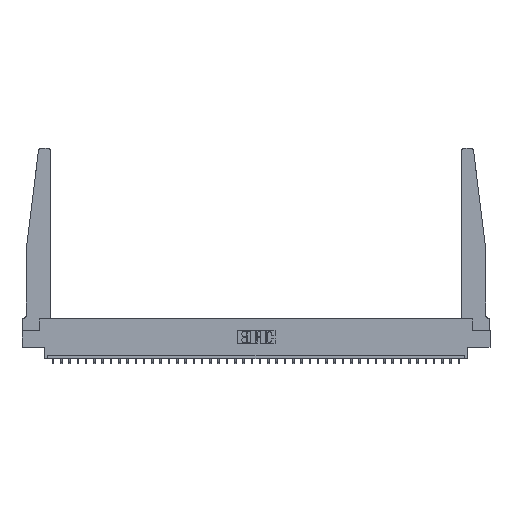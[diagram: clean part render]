
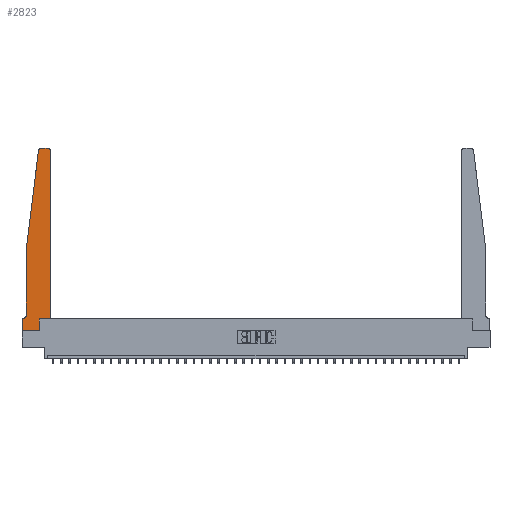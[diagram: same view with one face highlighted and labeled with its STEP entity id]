
A CAD part, top view. The second image highlights one B-rep face of the part: STEP entity #2823.
In plain terms, the highlighted planar face has unit normal (0, 0, 1).
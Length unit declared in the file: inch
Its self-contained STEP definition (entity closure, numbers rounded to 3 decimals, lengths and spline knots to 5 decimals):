
#106 = VERTEX_POINT ( 'NONE', #21183 ) ;
#502 = CARTESIAN_POINT ( 'NONE',  ( 0.2605, 0., 0.37 ) ) ;
#617 = ORIENTED_EDGE ( 'NONE', *, *, #6288, .T. ) ;
#631 = LINE ( 'NONE', #19562, #21369 ) ;
#884 = VECTOR ( 'NONE', #17345, 39.37008 ) ;
#1055 = CARTESIAN_POINT ( 'NONE',  ( 0.2605, 0.18, 0.37 ) ) ;
#1142 = ORIENTED_EDGE ( 'NONE', *, *, #24729, .T. ) ;
#1410 = CARTESIAN_POINT ( 'NONE',  ( 0.25, 2.75, 0.37 ) ) ;
#1413 = VECTOR ( 'NONE', #12961, 39.37008 ) ;
#2285 = ORIENTED_EDGE ( 'NONE', *, *, #34943, .T. ) ;
#2823 = ADVANCED_FACE ( 'NONE', ( #4828 ), #4085, .T. ) ;
#2883 = EDGE_CURVE ( 'NONE', #24931, #31924, #31074, .T. ) ;
#3437 = EDGE_CURVE ( 'NONE', #21624, #19020, #34818, .T. ) ;
#4085 = PLANE ( 'NONE',  #16069 ) ;
#4260 = VERTEX_POINT ( 'NONE', #10631 ) ;
#4573 = CARTESIAN_POINT ( 'NONE',  ( 0.065, 1.25, 0.37 ) ) ;
#4828 = FACE_OUTER_BOUND ( 'NONE', #7690, .T. ) ;
#5713 = VECTOR ( 'NONE', #20335, 39.37008 ) ;
#6008 = AXIS2_PLACEMENT_3D ( 'NONE', #9923, #28837, #12650 ) ;
#6239 = ORIENTED_EDGE ( 'NONE', *, *, #30972, .T. ) ;
#6288 = EDGE_CURVE ( 'NONE', #31924, #32049, #16930, .T. ) ;
#7283 = DIRECTION ( 'NONE',  ( -0.122, -0.992, 0. ) ) ;
#7435 = AXIS2_PLACEMENT_3D ( 'NONE', #12800, #31715, #15513 ) ;
#7573 = ORIENTED_EDGE ( 'NONE', *, *, #24124, .T. ) ;
#7690 = EDGE_LOOP ( 'NONE', ( #17055, #8442, #12728, #23685, #7573, #6239, #21444, #23729, #617, #2285, #1142, #27876 ) ) ;
#7839 = AXIS2_PLACEMENT_3D ( 'NONE', #31916, #15717, #34592 ) ;
#8350 = DIRECTION ( 'NONE',  ( -1., 0., 0. ) ) ;
#8442 = ORIENTED_EDGE ( 'NONE', *, *, #3437, .T. ) ;
#8556 = LINE ( 'NONE', #18305, #1413 ) ;
#8745 = DIRECTION ( 'NONE',  ( 0., -1., 0. ) ) ;
#9923 = CARTESIAN_POINT ( 'NONE',  ( 0.015, 0.2375, 0.37 ) ) ;
#10631 = CARTESIAN_POINT ( 'NONE',  ( 0.065, 0.2375, 0.37 ) ) ;
#11408 = LINE ( 'NONE', #24056, #18614 ) ;
#12240 = DIRECTION ( 'NONE',  ( 1., 0., 0. ) ) ;
#12650 = DIRECTION ( 'NONE',  ( -1., 0., 0. ) ) ;
#12728 = ORIENTED_EDGE ( 'NONE', *, *, #22366, .T. ) ;
#12782 = VERTEX_POINT ( 'NONE', #22865 ) ;
#12800 = CARTESIAN_POINT ( 'NONE',  ( 0.27653, 2.72, 0.37 ) ) ;
#12961 = DIRECTION ( 'NONE',  ( 0., 1., 0. ) ) ;
#13389 = LINE ( 'NONE', #32881, #21485 ) ;
#13698 = CIRCLE ( 'NONE', #7839, 0.03 ) ;
#14226 = CARTESIAN_POINT ( 'NONE',  ( 0., 0., 0.37 ) ) ;
#14302 = VERTEX_POINT ( 'NONE', #27363 ) ;
#15513 = DIRECTION ( 'NONE',  ( 1., 0., 0. ) ) ;
#15544 = LINE ( 'NONE', #4573, #28245 ) ;
#15635 = VERTEX_POINT ( 'NONE', #25544 ) ;
#15717 = DIRECTION ( 'NONE',  ( 0., 0., 1. ) ) ;
#15870 = LINE ( 'NONE', #24571, #30239 ) ;
#16069 = AXIS2_PLACEMENT_3D ( 'NONE', #23030, #28447, #12240 ) ;
#16695 = DIRECTION ( 'NONE',  ( 0., -1., 0. ) ) ;
#16930 = LINE ( 'NONE', #33522, #884 ) ;
#17055 = ORIENTED_EDGE ( 'NONE', *, *, #18005, .T. ) ;
#17345 = DIRECTION ( 'NONE',  ( 0., 1., 0. ) ) ;
#18005 = EDGE_CURVE ( 'NONE', #106, #21624, #18450, .T. ) ;
#18305 = CARTESIAN_POINT ( 'NONE',  ( 0.425, 0.18, 0.37 ) ) ;
#18450 = LINE ( 'NONE', #1410, #5713 ) ;
#18614 = VECTOR ( 'NONE', #34869, 39.37008 ) ;
#18995 = EDGE_CURVE ( 'NONE', #15635, #24931, #631, .T. ) ;
#19020 = VERTEX_POINT ( 'NONE', #22400 ) ;
#19562 = CARTESIAN_POINT ( 'NONE',  ( 0., 0., 0.37 ) ) ;
#20335 = DIRECTION ( 'NONE',  ( -1., 0., 0. ) ) ;
#21183 = CARTESIAN_POINT ( 'NONE',  ( 0.395, 2.75, 0.37 ) ) ;
#21369 = VECTOR ( 'NONE', #8745, 39.37008 ) ;
#21444 = ORIENTED_EDGE ( 'NONE', *, *, #18995, .T. ) ;
#21485 = VECTOR ( 'NONE', #16695, 39.37008 ) ;
#21624 = VERTEX_POINT ( 'NONE', #23234 ) ;
#22366 = EDGE_CURVE ( 'NONE', #19020, #26341, #15544, .T. ) ;
#22400 = CARTESIAN_POINT ( 'NONE',  ( 0.24675, 2.72367, 0.37 ) ) ;
#22652 = VERTEX_POINT ( 'NONE', #25281 ) ;
#22865 = CARTESIAN_POINT ( 'NONE',  ( 0.425, 2.72, 0.37 ) ) ;
#23030 = CARTESIAN_POINT ( 'NONE',  ( 0., 0.1875, 0.37 ) ) ;
#23234 = CARTESIAN_POINT ( 'NONE',  ( 0.27653, 2.75, 0.37 ) ) ;
#23685 = ORIENTED_EDGE ( 'NONE', *, *, #23812, .T. ) ;
#23729 = ORIENTED_EDGE ( 'NONE', *, *, #2883, .T. ) ;
#23812 = EDGE_CURVE ( 'NONE', #26341, #4260, #13389, .T. ) ;
#23928 = VECTOR ( 'NONE', #26064, 39.37008 ) ;
#24056 = CARTESIAN_POINT ( 'NONE',  ( 0.425, 0.18, 0.37 ) ) ;
#24124 = EDGE_CURVE ( 'NONE', #4260, #22652, #28087, .T. ) ;
#24166 = EDGE_CURVE ( 'NONE', #12782, #106, #13698, .T. ) ;
#24571 = CARTESIAN_POINT ( 'NONE',  ( 0.065, 0.1875, 0.37 ) ) ;
#24729 = EDGE_CURVE ( 'NONE', #14302, #12782, #8556, .T. ) ;
#24931 = VERTEX_POINT ( 'NONE', #14226 ) ;
#25281 = CARTESIAN_POINT ( 'NONE',  ( 0.015, 0.1875, 0.37 ) ) ;
#25544 = CARTESIAN_POINT ( 'NONE',  ( 0., 0.1875, 0.37 ) ) ;
#26064 = DIRECTION ( 'NONE',  ( 1., 0., 0. ) ) ;
#26341 = VERTEX_POINT ( 'NONE', #33606 ) ;
#27363 = CARTESIAN_POINT ( 'NONE',  ( 0.425, 0.18, 0.37 ) ) ;
#27876 = ORIENTED_EDGE ( 'NONE', *, *, #24166, .T. ) ;
#28087 = CIRCLE ( 'NONE', #6008, 0.05 ) ;
#28245 = VECTOR ( 'NONE', #7283, 39.37008 ) ;
#28447 = DIRECTION ( 'NONE',  ( 0., 0., 1. ) ) ;
#28781 = CARTESIAN_POINT ( 'NONE',  ( 0., 0., 0.37 ) ) ;
#28837 = DIRECTION ( 'NONE',  ( 0., 0., -1. ) ) ;
#30239 = VECTOR ( 'NONE', #8350, 39.37008 ) ;
#30972 = EDGE_CURVE ( 'NONE', #22652, #15635, #15870, .T. ) ;
#31074 = LINE ( 'NONE', #28781, #23928 ) ;
#31715 = DIRECTION ( 'NONE',  ( 0., 0., 1. ) ) ;
#31916 = CARTESIAN_POINT ( 'NONE',  ( 0.395, 2.72, 0.37 ) ) ;
#31924 = VERTEX_POINT ( 'NONE', #502 ) ;
#32049 = VERTEX_POINT ( 'NONE', #1055 ) ;
#32881 = CARTESIAN_POINT ( 'NONE',  ( 0.065, 1.25, 0.37 ) ) ;
#33522 = CARTESIAN_POINT ( 'NONE',  ( 0.2605, 0.18, 0.37 ) ) ;
#33606 = CARTESIAN_POINT ( 'NONE',  ( 0.065, 1.25, 0.37 ) ) ;
#34592 = DIRECTION ( 'NONE',  ( 1., 0., 0. ) ) ;
#34818 = CIRCLE ( 'NONE', #7435, 0.03 ) ;
#34869 = DIRECTION ( 'NONE',  ( 1., 0., 0. ) ) ;
#34943 = EDGE_CURVE ( 'NONE', #32049, #14302, #11408, .T. ) ;
